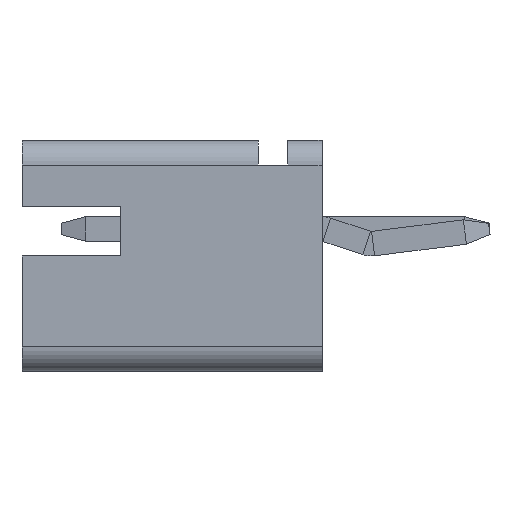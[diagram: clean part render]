
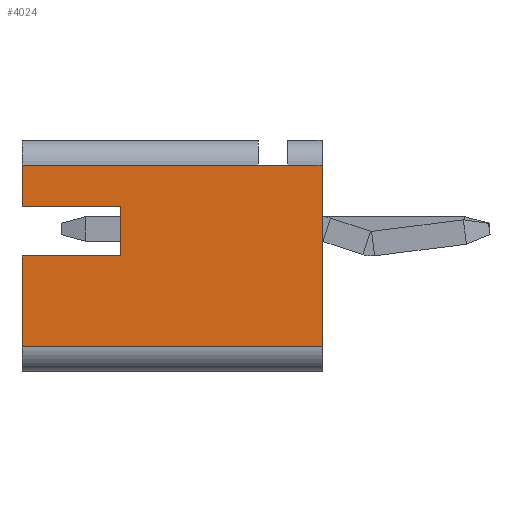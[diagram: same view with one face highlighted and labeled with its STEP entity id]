
A CAD part, left-side view. The second image highlights one B-rep face of the part: STEP entity #4024.
In plain terms, the highlighted planar face has unit normal (-1, 0, 0).
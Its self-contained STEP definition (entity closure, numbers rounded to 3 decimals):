
#64 = PLANE ( 'NONE',  #4279 ) ;
#75 = CARTESIAN_POINT ( 'NONE',  ( -2., 1.3, 1.3 ) ) ;
#89 = EDGE_CURVE ( 'NONE', #568, #3598, #4687, .T. ) ;
#143 = CARTESIAN_POINT ( 'NONE',  ( -2., 0., -2.4 ) ) ;
#202 = EDGE_CURVE ( 'NONE', #4533, #2481, #4411, .T. ) ;
#462 = LINE ( 'NONE', #1196, #4662 ) ;
#568 = VERTEX_POINT ( 'NONE', #1651 ) ;
#574 = CARTESIAN_POINT ( 'NONE',  ( -2., 0.7, 1.3 ) ) ;
#692 = CARTESIAN_POINT ( 'NONE',  ( -2., 0., 1.3 ) ) ;
#822 = FACE_OUTER_BOUND ( 'NONE', #5026, .T. ) ;
#888 = ORIENTED_EDGE ( 'NONE', *, *, #1629, .T. ) ;
#897 = ORIENTED_EDGE ( 'NONE', *, *, #4262, .F. ) ;
#944 = VERTEX_POINT ( 'NONE', #2734 ) ;
#971 = DIRECTION ( 'NONE',  ( 0., -1., 0. ) ) ;
#1172 = ORIENTED_EDGE ( 'NONE', *, *, #4505, .F. ) ;
#1196 = CARTESIAN_POINT ( 'NONE',  ( -2., 6.1, 1.8 ) ) ;
#1303 = ORIENTED_EDGE ( 'NONE', *, *, #3712, .F. ) ;
#1341 = DIRECTION ( 'NONE',  ( 0., -1., 0. ) ) ;
#1426 = VECTOR ( 'NONE', #3761, 1000. ) ;
#1435 = EDGE_CURVE ( 'NONE', #2997, #4533, #4213, .T. ) ;
#1490 = LINE ( 'NONE', #143, #5279 ) ;
#1629 = EDGE_CURVE ( 'NONE', #2997, #5643, #1490, .T. ) ;
#1651 = CARTESIAN_POINT ( 'NONE',  ( -2., 1.3, 1.3 ) ) ;
#1665 = DIRECTION ( 'NONE',  ( 0., 0., 1. ) ) ;
#1676 = CARTESIAN_POINT ( 'NONE',  ( -2., 6.1, -0.55 ) ) ;
#1708 = CARTESIAN_POINT ( 'NONE',  ( -2., 0., 1.8 ) ) ;
#1740 = ORIENTED_EDGE ( 'NONE', *, *, #4838, .F. ) ;
#1757 = VECTOR ( 'NONE', #1341, 1000. ) ;
#1883 = DIRECTION ( 'NONE',  ( 1., 0., 0. ) ) ;
#1941 = EDGE_CURVE ( 'NONE', #944, #5643, #5202, .T. ) ;
#2467 = CARTESIAN_POINT ( 'NONE',  ( -2., 6.1, -0.55 ) ) ;
#2481 = VERTEX_POINT ( 'NONE', #3204 ) ;
#2652 = LINE ( 'NONE', #75, #5377 ) ;
#2734 = CARTESIAN_POINT ( 'NONE',  ( -2., 0., 1.3 ) ) ;
#2841 = VECTOR ( 'NONE', #3481, 1000. ) ;
#2924 = LINE ( 'NONE', #5229, #3536 ) ;
#2997 = VERTEX_POINT ( 'NONE', #3880 ) ;
#3052 = CARTESIAN_POINT ( 'NONE',  ( -2., 4.1, 0.45 ) ) ;
#3094 = CARTESIAN_POINT ( 'NONE',  ( -2., 6.1, -0.55 ) ) ;
#3204 = CARTESIAN_POINT ( 'NONE',  ( -2., 4.1, -0.55 ) ) ;
#3259 = VERTEX_POINT ( 'NONE', #574 ) ;
#3294 = VECTOR ( 'NONE', #3944, 1000. ) ;
#3313 = DIRECTION ( 'NONE',  ( 0., -1., 0. ) ) ;
#3374 = CARTESIAN_POINT ( 'NONE',  ( -2., 6.1, 0.45 ) ) ;
#3380 = DIRECTION ( 'NONE',  ( 0., 1., 0. ) ) ;
#3481 = DIRECTION ( 'NONE',  ( 0., 0., 1. ) ) ;
#3525 = LINE ( 'NONE', #5553, #1426 ) ;
#3536 = VECTOR ( 'NONE', #3380, 1000. ) ;
#3598 = VERTEX_POINT ( 'NONE', #5223 ) ;
#3712 = EDGE_CURVE ( 'NONE', #568, #3259, #2652, .T. ) ;
#3761 = DIRECTION ( 'NONE',  ( 0., 1., 0. ) ) ;
#3789 = ORIENTED_EDGE ( 'NONE', *, *, #1435, .F. ) ;
#3817 = DIRECTION ( 'NONE',  ( 0., 1., 0. ) ) ;
#3880 = CARTESIAN_POINT ( 'NONE',  ( -2., 6.1, -2.4 ) ) ;
#3944 = DIRECTION ( 'NONE',  ( 0., 0., -1. ) ) ;
#3975 = CARTESIAN_POINT ( 'NONE',  ( -2., 0., -2.4 ) ) ;
#4024 = ADVANCED_FACE ( 'NONE', ( #822 ), #64, .F. ) ;
#4034 = LINE ( 'NONE', #3052, #2841 ) ;
#4109 = CARTESIAN_POINT ( 'NONE',  ( -2., 4.1, 0.45 ) ) ;
#4174 = ORIENTED_EDGE ( 'NONE', *, *, #89, .T. ) ;
#4213 = LINE ( 'NONE', #1676, #5535 ) ;
#4262 = EDGE_CURVE ( 'NONE', #4865, #4473, #2924, .T. ) ;
#4279 = AXIS2_PLACEMENT_3D ( 'NONE', #5069, #1883, #5003 ) ;
#4411 = LINE ( 'NONE', #3094, #1757 ) ;
#4473 = VERTEX_POINT ( 'NONE', #3374 ) ;
#4505 = EDGE_CURVE ( 'NONE', #4473, #3598, #462, .T. ) ;
#4533 = VERTEX_POINT ( 'NONE', #2467 ) ;
#4662 = VECTOR ( 'NONE', #1665, 1000. ) ;
#4687 = LINE ( 'NONE', #692, #5744 ) ;
#4770 = ORIENTED_EDGE ( 'NONE', *, *, #5390, .T. ) ;
#4838 = EDGE_CURVE ( 'NONE', #2481, #4865, #4034, .T. ) ;
#4865 = VERTEX_POINT ( 'NONE', #4109 ) ;
#4962 = ORIENTED_EDGE ( 'NONE', *, *, #1941, .F. ) ;
#5003 = DIRECTION ( 'NONE',  ( 0., 0., -1. ) ) ;
#5026 = EDGE_LOOP ( 'NONE', ( #3789, #888, #4962, #4770, #1303, #4174, #1172, #897, #1740, #5587 ) ) ;
#5069 = CARTESIAN_POINT ( 'NONE',  ( -2., 0., 0. ) ) ;
#5202 = LINE ( 'NONE', #1708, #3294 ) ;
#5223 = CARTESIAN_POINT ( 'NONE',  ( -2., 6.1, 1.3 ) ) ;
#5229 = CARTESIAN_POINT ( 'NONE',  ( -2., 6.1, 0.45 ) ) ;
#5255 = DIRECTION ( 'NONE',  ( 0., 0., 1. ) ) ;
#5279 = VECTOR ( 'NONE', #3313, 1000. ) ;
#5377 = VECTOR ( 'NONE', #971, 1000. ) ;
#5390 = EDGE_CURVE ( 'NONE', #944, #3259, #3525, .T. ) ;
#5535 = VECTOR ( 'NONE', #5255, 1000. ) ;
#5553 = CARTESIAN_POINT ( 'NONE',  ( -2., 0., 1.3 ) ) ;
#5587 = ORIENTED_EDGE ( 'NONE', *, *, #202, .F. ) ;
#5643 = VERTEX_POINT ( 'NONE', #3975 ) ;
#5744 = VECTOR ( 'NONE', #3817, 1000. ) ;
